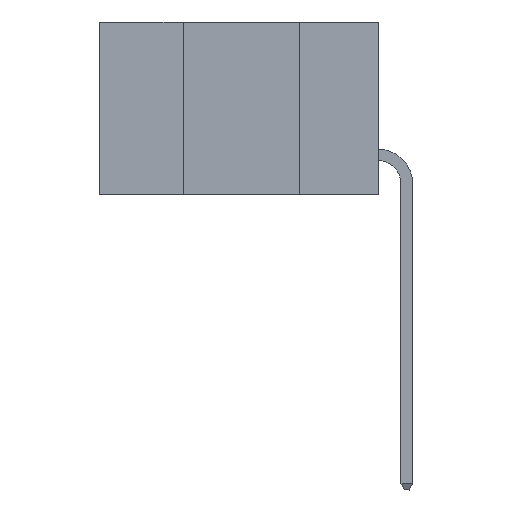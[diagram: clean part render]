
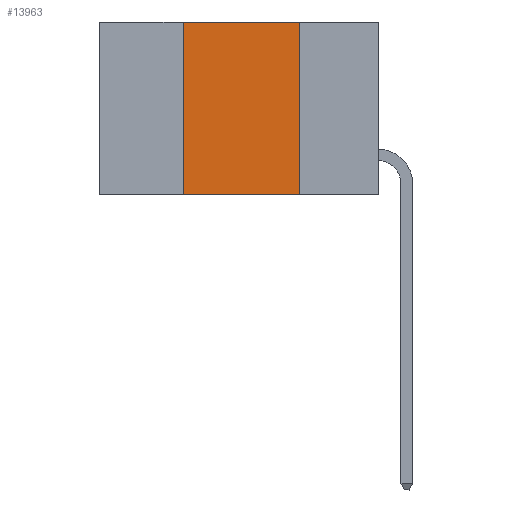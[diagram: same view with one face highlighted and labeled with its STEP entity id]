
A CAD part, left-side view. The second image highlights one B-rep face of the part: STEP entity #13963.
In plain terms, the highlighted planar face has unit normal (-1, 0, 0).
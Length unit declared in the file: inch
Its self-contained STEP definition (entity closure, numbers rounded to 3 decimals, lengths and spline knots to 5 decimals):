
#122 = EDGE_CURVE ( 'NONE', #9701, #3485, #12588, .T. ) ;
#127 = CARTESIAN_POINT ( 'NONE',  ( 0., 0.42, -0.37 ) ) ;
#803 = CARTESIAN_POINT ( 'NONE',  ( 0., 0.6, 0. ) ) ;
#1508 = CARTESIAN_POINT ( 'NONE',  ( 0., 0.42, 0. ) ) ;
#1735 = VECTOR ( 'NONE', #3201, 39.37008 ) ;
#1737 = CARTESIAN_POINT ( 'NONE',  ( 0., 0.17, -0.37 ) ) ;
#2471 = ORIENTED_EDGE ( 'NONE', *, *, #122, .F. ) ;
#2614 = DIRECTION ( 'NONE',  ( 0., 0., -1. ) ) ;
#2982 = DIRECTION ( 'NONE',  ( 0., 0., -1. ) ) ;
#3058 = DIRECTION ( 'NONE',  ( 0., -1., 0. ) ) ;
#3201 = DIRECTION ( 'NONE',  ( 0., -1., 0. ) ) ;
#3485 = VERTEX_POINT ( 'NONE', #12885 ) ;
#3788 = PLANE ( 'NONE',  #14034 ) ;
#4306 = DIRECTION ( 'NONE',  ( 0., 0., 1. ) ) ;
#4345 = VECTOR ( 'NONE', #4306, 39.37008 ) ;
#4711 = VERTEX_POINT ( 'NONE', #5356 ) ;
#5174 = CARTESIAN_POINT ( 'NONE',  ( 0., 0.6, -0.37 ) ) ;
#5356 = CARTESIAN_POINT ( 'NONE',  ( 0., 0.17, -0.37 ) ) ;
#7542 = VECTOR ( 'NONE', #3058, 39.37008 ) ;
#7593 = LINE ( 'NONE', #5174, #7542 ) ;
#7894 = CARTESIAN_POINT ( 'NONE',  ( 0., 0.42, -0.37 ) ) ;
#8180 = EDGE_LOOP ( 'NONE', ( #8324, #2471, #13519, #8559 ) ) ;
#8324 = ORIENTED_EDGE ( 'NONE', *, *, #10479, .F. ) ;
#8527 = CARTESIAN_POINT ( 'NONE',  ( 0., 0.6, 0. ) ) ;
#8559 = ORIENTED_EDGE ( 'NONE', *, *, #10397, .T. ) ;
#9044 = LINE ( 'NONE', #7894, #4345 ) ;
#9701 = VERTEX_POINT ( 'NONE', #1508 ) ;
#10322 = VERTEX_POINT ( 'NONE', #127 ) ;
#10397 = EDGE_CURVE ( 'NONE', #10322, #4711, #7593, .T. ) ;
#10479 = EDGE_CURVE ( 'NONE', #3485, #4711, #12369, .T. ) ;
#12224 = VECTOR ( 'NONE', #2982, 39.37008 ) ;
#12369 = LINE ( 'NONE', #1737, #12224 ) ;
#12588 = LINE ( 'NONE', #803, #1735 ) ;
#12880 = EDGE_CURVE ( 'NONE', #10322, #9701, #9044, .T. ) ;
#12885 = CARTESIAN_POINT ( 'NONE',  ( 0., 0.17, 0. ) ) ;
#13228 = DIRECTION ( 'NONE',  ( 1., 0., 0. ) ) ;
#13519 = ORIENTED_EDGE ( 'NONE', *, *, #12880, .F. ) ;
#13963 = ADVANCED_FACE ( 'NONE', ( #14372 ), #3788, .F. ) ;
#14034 = AXIS2_PLACEMENT_3D ( 'NONE', #8527, #13228, #2614 ) ;
#14372 = FACE_OUTER_BOUND ( 'NONE', #8180, .T. ) ;
